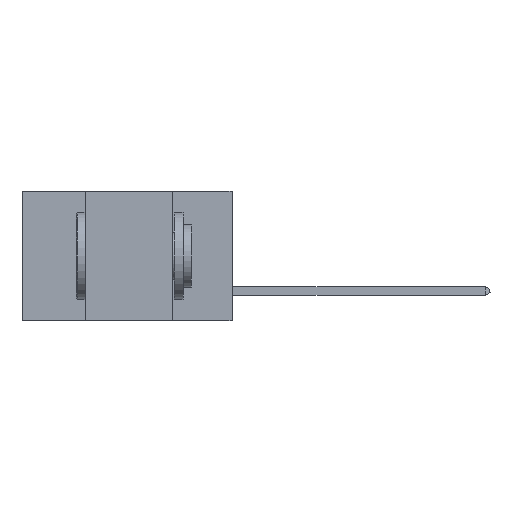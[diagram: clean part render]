
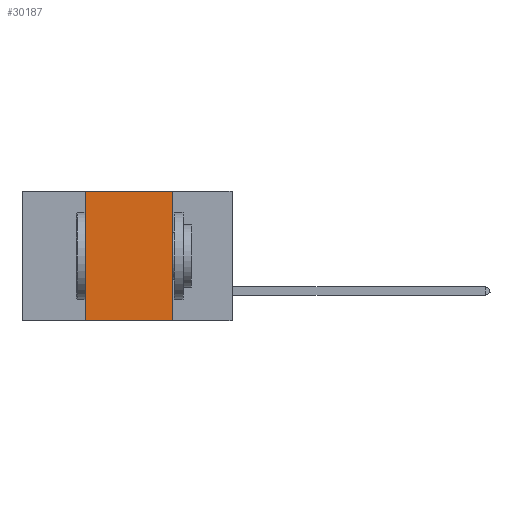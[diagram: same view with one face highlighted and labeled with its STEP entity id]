
A CAD part, left-side view. The second image highlights one B-rep face of the part: STEP entity #30187.
In plain terms, the highlighted planar face has unit normal (-1, 0, 0).
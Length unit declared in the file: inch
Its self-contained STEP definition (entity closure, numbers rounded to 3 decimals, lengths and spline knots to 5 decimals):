
#2168 = DIRECTION ( 'NONE',  ( 1., 0., 0. ) ) ;
#2830 = CARTESIAN_POINT ( 'NONE',  ( 0., 0.42, 0. ) ) ;
#7617 = EDGE_LOOP ( 'NONE', ( #44914, #18950, #31299, #12453 ) ) ;
#9124 = CARTESIAN_POINT ( 'NONE',  ( 0., 0.6, 0. ) ) ;
#12453 = ORIENTED_EDGE ( 'NONE', *, *, #20792, .T. ) ;
#13170 = DIRECTION ( 'NONE',  ( 0., 0., -1. ) ) ;
#13993 = DIRECTION ( 'NONE',  ( 0., -1., 0. ) ) ;
#17722 = CARTESIAN_POINT ( 'NONE',  ( 0., 0.17, 0. ) ) ;
#18950 = ORIENTED_EDGE ( 'NONE', *, *, #37283, .F. ) ;
#20452 = PLANE ( 'NONE',  #44124 ) ;
#20519 = DIRECTION ( 'NONE',  ( 0., -1., 0. ) ) ;
#20792 = EDGE_CURVE ( 'NONE', #22384, #42134, #29582, .T. ) ;
#22384 = VERTEX_POINT ( 'NONE', #43098 ) ;
#22680 = VECTOR ( 'NONE', #13993, 39.37008 ) ;
#24321 = FACE_OUTER_BOUND ( 'NONE', #7617, .T. ) ;
#27183 = EDGE_CURVE ( 'NONE', #22384, #36892, #39586, .T. ) ;
#27807 = LINE ( 'NONE', #36376, #43301 ) ;
#28853 = DIRECTION ( 'NONE',  ( 0., 0., -1. ) ) ;
#29582 = LINE ( 'NONE', #32859, #22680 ) ;
#30187 = ADVANCED_FACE ( 'NONE', ( #24321 ), #20452, .F. ) ;
#30335 = EDGE_CURVE ( 'NONE', #34215, #42134, #27807, .T. ) ;
#30463 = VECTOR ( 'NONE', #32075, 39.37008 ) ;
#31299 = ORIENTED_EDGE ( 'NONE', *, *, #27183, .F. ) ;
#32075 = DIRECTION ( 'NONE',  ( 0., 0., 1. ) ) ;
#32859 = CARTESIAN_POINT ( 'NONE',  ( 0., 0.6, -0.37 ) ) ;
#34215 = VERTEX_POINT ( 'NONE', #17722 ) ;
#36376 = CARTESIAN_POINT ( 'NONE',  ( 0., 0.17, 0. ) ) ;
#36892 = VERTEX_POINT ( 'NONE', #2830 ) ;
#37283 = EDGE_CURVE ( 'NONE', #36892, #34215, #41019, .T. ) ;
#39586 = LINE ( 'NONE', #46586, #30463 ) ;
#41019 = LINE ( 'NONE', #46464, #47398 ) ;
#42134 = VERTEX_POINT ( 'NONE', #44424 ) ;
#43098 = CARTESIAN_POINT ( 'NONE',  ( 0., 0.42, -0.37 ) ) ;
#43301 = VECTOR ( 'NONE', #28853, 39.37008 ) ;
#44124 = AXIS2_PLACEMENT_3D ( 'NONE', #9124, #2168, #13170 ) ;
#44424 = CARTESIAN_POINT ( 'NONE',  ( 0., 0.17, -0.37 ) ) ;
#44914 = ORIENTED_EDGE ( 'NONE', *, *, #30335, .F. ) ;
#46464 = CARTESIAN_POINT ( 'NONE',  ( 0., 0.6, 0. ) ) ;
#46586 = CARTESIAN_POINT ( 'NONE',  ( 0., 0.42, 0. ) ) ;
#47398 = VECTOR ( 'NONE', #20519, 39.37008 ) ;
